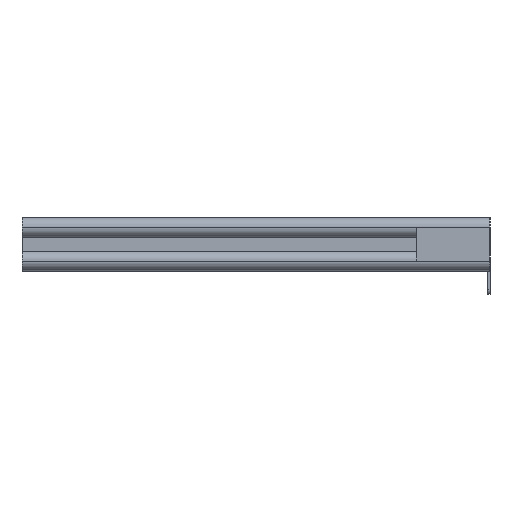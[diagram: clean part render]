
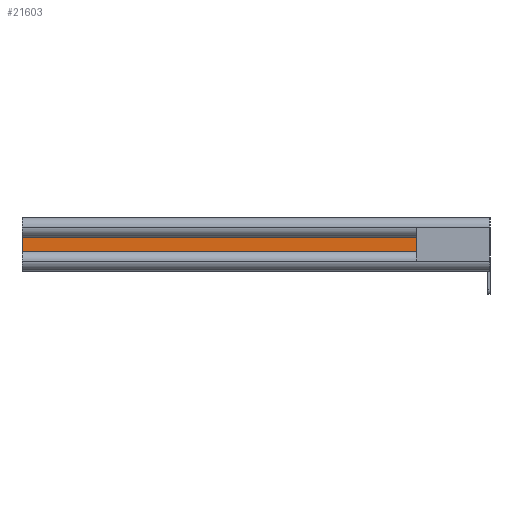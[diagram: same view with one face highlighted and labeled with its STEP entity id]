
A CAD part, left-side view. The second image highlights one B-rep face of the part: STEP entity #21603.
In plain terms, the highlighted planar face has unit normal (-1, 0, 0).
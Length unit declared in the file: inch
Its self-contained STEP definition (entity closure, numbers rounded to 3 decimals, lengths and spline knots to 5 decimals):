
#110 = EDGE_CURVE ( 'NONE', #19067, #13567, #3199, .T. ) ;
#242 = VERTEX_POINT ( 'NONE', #3168 ) ;
#658 = ORIENTED_EDGE ( 'NONE', *, *, #23406, .F. ) ;
#874 = CARTESIAN_POINT ( 'NONE',  ( 0.044, 0.37012, -0.0465 ) ) ;
#1258 = VECTOR ( 'NONE', #19279, 39.37008 ) ;
#1311 = CARTESIAN_POINT ( 'NONE',  ( 0.044, 0.37012, -0.0465 ) ) ;
#1417 = EDGE_CURVE ( 'NONE', #19067, #242, #6876, .T. ) ;
#2068 = LINE ( 'NONE', #874, #5887 ) ;
#3168 = CARTESIAN_POINT ( 'NONE',  ( 0.044, 3., 0.0465 ) ) ;
#3199 = LINE ( 'NONE', #22496, #12380 ) ;
#3245 = DIRECTION ( 'NONE',  ( 0., 0., -1. ) ) ;
#5887 = VECTOR ( 'NONE', #22692, 39.37008 ) ;
#6609 = ORIENTED_EDGE ( 'NONE', *, *, #1417, .T. ) ;
#6876 = LINE ( 'NONE', #17486, #20118 ) ;
#8241 = CARTESIAN_POINT ( 'NONE',  ( 0.044, 0.473, 0.0465 ) ) ;
#9971 = FACE_OUTER_BOUND ( 'NONE', #13170, .T. ) ;
#10248 = CARTESIAN_POINT ( 'NONE',  ( 0.044, 3., -0.0465 ) ) ;
#12380 = VECTOR ( 'NONE', #16988, 39.37008 ) ;
#13170 = EDGE_LOOP ( 'NONE', ( #6609, #17568, #658, #22706 ) ) ;
#13567 = VERTEX_POINT ( 'NONE', #22711 ) ;
#14197 = DIRECTION ( 'NONE',  ( 1., 0., 0. ) ) ;
#16451 = CARTESIAN_POINT ( 'NONE',  ( 0.044, 3., -0.0465 ) ) ;
#16988 = DIRECTION ( 'NONE',  ( 0., 0., -1. ) ) ;
#17486 = CARTESIAN_POINT ( 'NONE',  ( 0.044, 0.37012, 0.0465 ) ) ;
#17568 = ORIENTED_EDGE ( 'NONE', *, *, #20944, .T. ) ;
#18775 = VERTEX_POINT ( 'NONE', #16451 ) ;
#19067 = VERTEX_POINT ( 'NONE', #8241 ) ;
#19279 = DIRECTION ( 'NONE',  ( 0., 0., -1. ) ) ;
#20118 = VECTOR ( 'NONE', #20899, 39.37008 ) ;
#20605 = LINE ( 'NONE', #10248, #1258 ) ;
#20899 = DIRECTION ( 'NONE',  ( 0., 1., 0. ) ) ;
#20944 = EDGE_CURVE ( 'NONE', #242, #18775, #20605, .T. ) ;
#21603 = ADVANCED_FACE ( 'NONE', ( #9971 ), #23036, .F. ) ;
#21792 = AXIS2_PLACEMENT_3D ( 'NONE', #1311, #14197, #3245 ) ;
#22496 = CARTESIAN_POINT ( 'NONE',  ( 0.044, 0.473, -0.0465 ) ) ;
#22692 = DIRECTION ( 'NONE',  ( 0., 1., 0. ) ) ;
#22706 = ORIENTED_EDGE ( 'NONE', *, *, #110, .F. ) ;
#22711 = CARTESIAN_POINT ( 'NONE',  ( 0.044, 0.473, -0.0465 ) ) ;
#23036 = PLANE ( 'NONE',  #21792 ) ;
#23406 = EDGE_CURVE ( 'NONE', #13567, #18775, #2068, .T. ) ;
